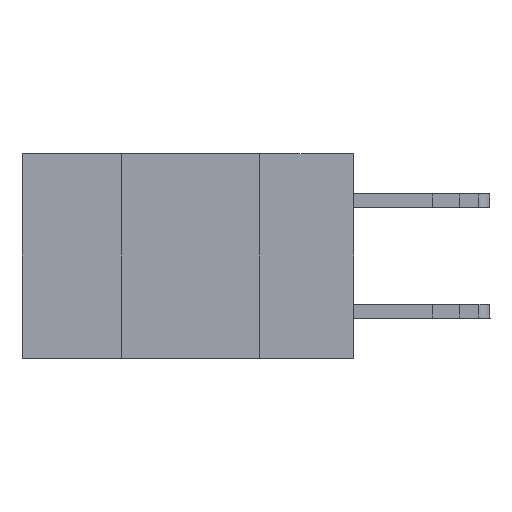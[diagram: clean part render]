
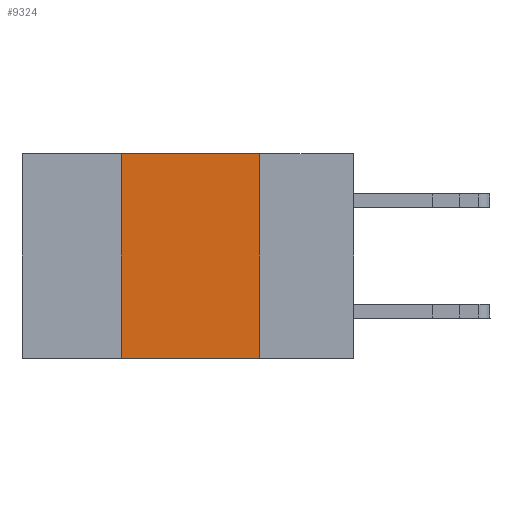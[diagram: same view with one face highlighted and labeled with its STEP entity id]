
A CAD part, left-side view. The second image highlights one B-rep face of the part: STEP entity #9324.
In plain terms, the highlighted planar face has unit normal (-1, 0, 0).
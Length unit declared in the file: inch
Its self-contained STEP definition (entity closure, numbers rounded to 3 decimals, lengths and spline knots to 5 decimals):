
#161 = VERTEX_POINT ( 'NONE', #5803 ) ;
#1211 = DIRECTION ( 'NONE',  ( 1., 0., 0. ) ) ;
#1429 = DIRECTION ( 'NONE',  ( 0., 0., -1. ) ) ;
#1758 = EDGE_CURVE ( 'NONE', #18910, #29599, #28905, .T. ) ;
#2279 = ORIENTED_EDGE ( 'NONE', *, *, #4784, .F. ) ;
#3890 = LINE ( 'NONE', #30640, #22596 ) ;
#4089 = FACE_OUTER_BOUND ( 'NONE', #12470, .T. ) ;
#4752 = DIRECTION ( 'NONE',  ( 0., -1., 0. ) ) ;
#4784 = EDGE_CURVE ( 'NONE', #13613, #29599, #3890, .T. ) ;
#4968 = CARTESIAN_POINT ( 'NONE',  ( 0., 0.6, -0.37 ) ) ;
#5803 = CARTESIAN_POINT ( 'NONE',  ( 0., 0.42, 0. ) ) ;
#6135 = DIRECTION ( 'NONE',  ( 0., 0., -1. ) ) ;
#7749 = AXIS2_PLACEMENT_3D ( 'NONE', #23322, #1211, #1429 ) ;
#9324 = ADVANCED_FACE ( 'NONE', ( #4089 ), #16063, .F. ) ;
#9875 = CARTESIAN_POINT ( 'NONE',  ( 0., 0.42, -0.37 ) ) ;
#11036 = VECTOR ( 'NONE', #16788, 39.37008 ) ;
#12470 = EDGE_LOOP ( 'NONE', ( #2279, #30245, #31208, #30554 ) ) ;
#13613 = VERTEX_POINT ( 'NONE', #15336 ) ;
#14715 = VECTOR ( 'NONE', #22639, 39.37008 ) ;
#15336 = CARTESIAN_POINT ( 'NONE',  ( 0., 0.17, 0. ) ) ;
#16063 = PLANE ( 'NONE',  #7749 ) ;
#16689 = CARTESIAN_POINT ( 'NONE',  ( 0., 0.42, 0. ) ) ;
#16788 = DIRECTION ( 'NONE',  ( 0., 0., 1. ) ) ;
#17884 = VECTOR ( 'NONE', #4752, 39.37008 ) ;
#18910 = VERTEX_POINT ( 'NONE', #9875 ) ;
#19733 = CARTESIAN_POINT ( 'NONE',  ( 0., 0.6, 0. ) ) ;
#20735 = CARTESIAN_POINT ( 'NONE',  ( 0., 0.17, -0.37 ) ) ;
#22596 = VECTOR ( 'NONE', #6135, 39.37008 ) ;
#22639 = DIRECTION ( 'NONE',  ( 0., -1., 0. ) ) ;
#23322 = CARTESIAN_POINT ( 'NONE',  ( 0., 0.6, 0. ) ) ;
#24005 = LINE ( 'NONE', #16689, #11036 ) ;
#24040 = EDGE_CURVE ( 'NONE', #18910, #161, #24005, .T. ) ;
#26909 = LINE ( 'NONE', #19733, #14715 ) ;
#28905 = LINE ( 'NONE', #4968, #17884 ) ;
#29599 = VERTEX_POINT ( 'NONE', #20735 ) ;
#30245 = ORIENTED_EDGE ( 'NONE', *, *, #31170, .F. ) ;
#30554 = ORIENTED_EDGE ( 'NONE', *, *, #1758, .T. ) ;
#30640 = CARTESIAN_POINT ( 'NONE',  ( 0., 0.17, 0. ) ) ;
#31170 = EDGE_CURVE ( 'NONE', #161, #13613, #26909, .T. ) ;
#31208 = ORIENTED_EDGE ( 'NONE', *, *, #24040, .F. ) ;
